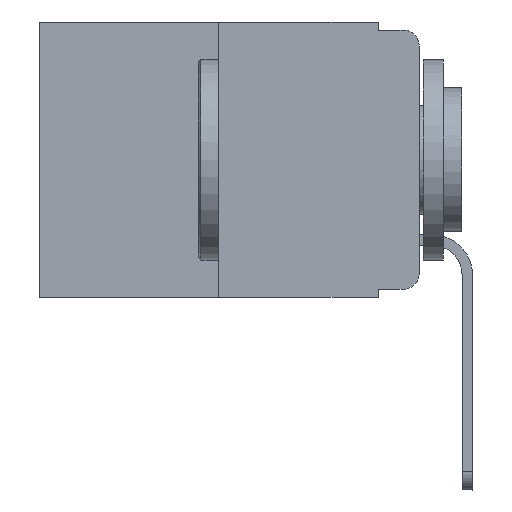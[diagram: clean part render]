
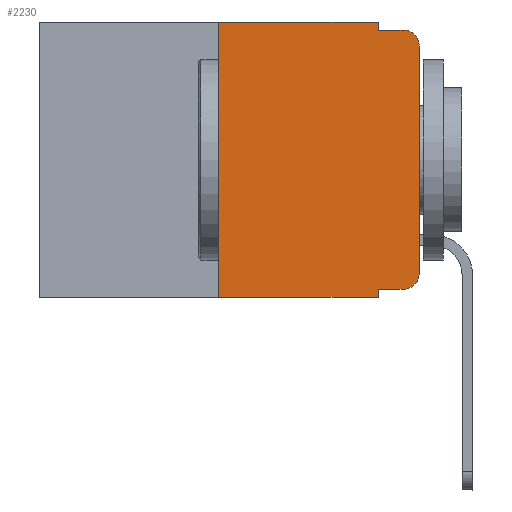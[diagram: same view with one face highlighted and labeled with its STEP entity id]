
A CAD part, left-side view. The second image highlights one B-rep face of the part: STEP entity #2230.
In plain terms, the highlighted planar face has unit normal (-1, 0, 0).
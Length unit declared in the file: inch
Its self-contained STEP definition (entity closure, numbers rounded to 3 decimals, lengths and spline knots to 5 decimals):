
#16 = VERTEX_POINT ( 'NONE', #20161 ) ;
#230 = CARTESIAN_POINT ( 'NONE',  ( 0., 0.25, 0. ) ) ;
#436 = LINE ( 'NONE', #10566, #8478 ) ;
#917 = DIRECTION ( 'NONE',  ( 0., -1., 0. ) ) ;
#1149 = VECTOR ( 'NONE', #2966, 39.37008 ) ;
#1424 = CARTESIAN_POINT ( 'NONE',  ( 0., 0.051, 0. ) ) ;
#1684 = EDGE_CURVE ( 'NONE', #8579, #3524, #10361, .T. ) ;
#1770 = CARTESIAN_POINT ( 'NONE',  ( 0., 0., -0.03 ) ) ;
#2230 = ADVANCED_FACE ( 'NONE', ( #21661 ), #3066, .F. ) ;
#2528 = CARTESIAN_POINT ( 'NONE',  ( 0., 0., 0. ) ) ;
#2595 = VERTEX_POINT ( 'NONE', #4466 ) ;
#2682 = VERTEX_POINT ( 'NONE', #21411 ) ;
#2966 = DIRECTION ( 'NONE',  ( 0., 0., -1. ) ) ;
#3066 = PLANE ( 'NONE',  #11659 ) ;
#3366 = EDGE_CURVE ( 'NONE', #16, #8579, #7561, .T. ) ;
#3524 = VERTEX_POINT ( 'NONE', #15143 ) ;
#3658 = AXIS2_PLACEMENT_3D ( 'NONE', #18868, #3914, #10507 ) ;
#3754 = ORIENTED_EDGE ( 'NONE', *, *, #10716, .T. ) ;
#3756 = VERTEX_POINT ( 'NONE', #9397 ) ;
#3882 = DIRECTION ( 'NONE',  ( 0., 0., 1. ) ) ;
#3914 = DIRECTION ( 'NONE',  ( -1., 0., 0. ) ) ;
#3969 = DIRECTION ( 'NONE',  ( 0., -1., 0. ) ) ;
#4466 = CARTESIAN_POINT ( 'NONE',  ( 0., 0.051, -0.343 ) ) ;
#4821 = DIRECTION ( 'NONE',  ( 0., 0., -1. ) ) ;
#5411 = DIRECTION ( 'NONE',  ( 0., -1., 0. ) ) ;
#5573 = VECTOR ( 'NONE', #917, 39.37008 ) ;
#5669 = ORIENTED_EDGE ( 'NONE', *, *, #18153, .F. ) ;
#5945 = CARTESIAN_POINT ( 'NONE',  ( 0., 0.02, -0.03 ) ) ;
#6030 = DIRECTION ( 'NONE',  ( 0., 0., 1. ) ) ;
#6370 = VECTOR ( 'NONE', #6030, 39.37008 ) ;
#6472 = LINE ( 'NONE', #13207, #7817 ) ;
#6613 = ORIENTED_EDGE ( 'NONE', *, *, #11681, .T. ) ;
#6844 = AXIS2_PLACEMENT_3D ( 'NONE', #5945, #14418, #21139 ) ;
#7150 = CARTESIAN_POINT ( 'NONE',  ( 0., 0.051, -0.333 ) ) ;
#7561 = LINE ( 'NONE', #2528, #6370 ) ;
#7770 = CARTESIAN_POINT ( 'NONE',  ( 0., 0.051, 0. ) ) ;
#7817 = VECTOR ( 'NONE', #4821, 39.37008 ) ;
#7981 = LINE ( 'NONE', #9749, #18094 ) ;
#8478 = VECTOR ( 'NONE', #3969, 39.37008 ) ;
#8579 = VERTEX_POINT ( 'NONE', #1770 ) ;
#9397 = CARTESIAN_POINT ( 'NONE',  ( 0., 0.051, -0.01 ) ) ;
#9721 = ORIENTED_EDGE ( 'NONE', *, *, #14659, .F. ) ;
#9749 = CARTESIAN_POINT ( 'NONE',  ( 0., 0.473, -0.343 ) ) ;
#9759 = DIRECTION ( 'NONE',  ( 0., 0., -1. ) ) ;
#9915 = VECTOR ( 'NONE', #5411, 39.37008 ) ;
#9949 = CIRCLE ( 'NONE', #3658, 0.02 ) ;
#9973 = CARTESIAN_POINT ( 'NONE',  ( 0., 0.473, 0. ) ) ;
#10088 = EDGE_CURVE ( 'NONE', #19090, #2595, #6472, .T. ) ;
#10144 = VECTOR ( 'NONE', #3882, 39.37008 ) ;
#10361 = CIRCLE ( 'NONE', #6844, 0.02 ) ;
#10507 = DIRECTION ( 'NONE',  ( 0., 0., -1. ) ) ;
#10566 = CARTESIAN_POINT ( 'NONE',  ( 0., 0.473, 0. ) ) ;
#10716 = EDGE_CURVE ( 'NONE', #18706, #16, #9949, .T. ) ;
#11416 = DIRECTION ( 'NONE',  ( 0., -1., 0. ) ) ;
#11659 = AXIS2_PLACEMENT_3D ( 'NONE', #9973, #13295, #9759 ) ;
#11681 = EDGE_CURVE ( 'NONE', #21315, #2595, #7981, .T. ) ;
#11730 = CARTESIAN_POINT ( 'NONE',  ( 0., 0.02, -0.333 ) ) ;
#12017 = LINE ( 'NONE', #230, #10144 ) ;
#12737 = CARTESIAN_POINT ( 'NONE',  ( 0., 0.25, -0.343 ) ) ;
#12833 = ORIENTED_EDGE ( 'NONE', *, *, #1684, .T. ) ;
#13207 = CARTESIAN_POINT ( 'NONE',  ( 0., 0.051, 0. ) ) ;
#13295 = DIRECTION ( 'NONE',  ( 1., 0., 0. ) ) ;
#13781 = LINE ( 'NONE', #7150, #9915 ) ;
#13972 = ORIENTED_EDGE ( 'NONE', *, *, #14909, .F. ) ;
#14418 = DIRECTION ( 'NONE',  ( -1., 0., 0. ) ) ;
#14587 = ORIENTED_EDGE ( 'NONE', *, *, #17850, .F. ) ;
#14659 = EDGE_CURVE ( 'NONE', #3756, #3524, #15992, .T. ) ;
#14909 = EDGE_CURVE ( 'NONE', #21315, #2682, #12017, .T. ) ;
#15143 = CARTESIAN_POINT ( 'NONE',  ( 0., 0.02, -0.01 ) ) ;
#15197 = ORIENTED_EDGE ( 'NONE', *, *, #3366, .T. ) ;
#15992 = LINE ( 'NONE', #19637, #5573 ) ;
#16144 = LINE ( 'NONE', #7770, #1149 ) ;
#16519 = CARTESIAN_POINT ( 'NONE',  ( 0., 0.051, -0.333 ) ) ;
#17323 = ORIENTED_EDGE ( 'NONE', *, *, #10088, .F. ) ;
#17375 = EDGE_LOOP ( 'NONE', ( #15197, #12833, #9721, #5669, #14587, #13972, #6613, #17323, #20001, #3754 ) ) ;
#17850 = EDGE_CURVE ( 'NONE', #2682, #20031, #436, .T. ) ;
#18094 = VECTOR ( 'NONE', #11416, 39.37008 ) ;
#18153 = EDGE_CURVE ( 'NONE', #20031, #3756, #16144, .T. ) ;
#18706 = VERTEX_POINT ( 'NONE', #11730 ) ;
#18868 = CARTESIAN_POINT ( 'NONE',  ( 0., 0.02, -0.313 ) ) ;
#19090 = VERTEX_POINT ( 'NONE', #16519 ) ;
#19272 = EDGE_CURVE ( 'NONE', #19090, #18706, #13781, .T. ) ;
#19637 = CARTESIAN_POINT ( 'NONE',  ( 0., 0.051, -0.01 ) ) ;
#20001 = ORIENTED_EDGE ( 'NONE', *, *, #19272, .T. ) ;
#20031 = VERTEX_POINT ( 'NONE', #1424 ) ;
#20161 = CARTESIAN_POINT ( 'NONE',  ( 0., 0., -0.313 ) ) ;
#21139 = DIRECTION ( 'NONE',  ( 0., 0., -1. ) ) ;
#21315 = VERTEX_POINT ( 'NONE', #12737 ) ;
#21411 = CARTESIAN_POINT ( 'NONE',  ( 0., 0.25, 0. ) ) ;
#21661 = FACE_OUTER_BOUND ( 'NONE', #17375, .T. ) ;
